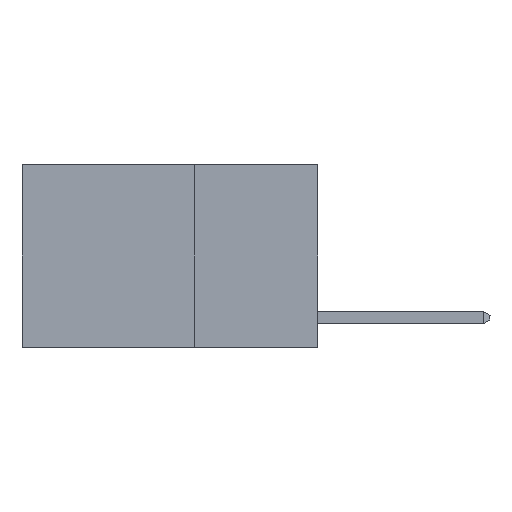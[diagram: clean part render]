
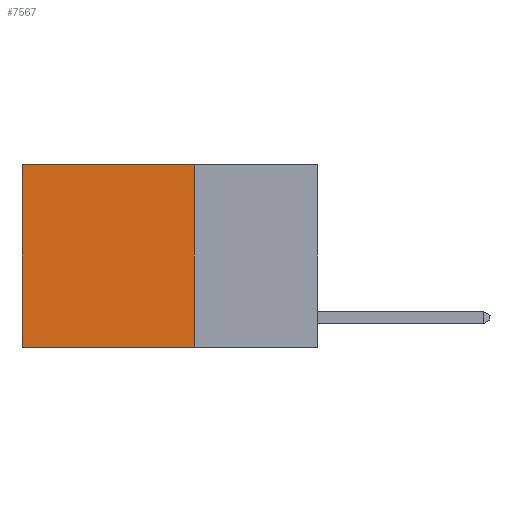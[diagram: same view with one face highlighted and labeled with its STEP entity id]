
A CAD part, left-side view. The second image highlights one B-rep face of the part: STEP entity #7567.
In plain terms, the highlighted planar face has unit normal (-1, 0, 0).
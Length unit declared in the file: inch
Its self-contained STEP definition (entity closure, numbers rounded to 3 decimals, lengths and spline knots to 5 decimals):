
#703 = AXIS2_PLACEMENT_3D ( 'NONE', #1785, #10758, #3123 ) ;
#1694 = EDGE_CURVE ( 'NONE', #4359, #4167, #3257, .T. ) ;
#1785 = CARTESIAN_POINT ( 'NONE',  ( 0.2625, 0.25, 0. ) ) ;
#1978 = CARTESIAN_POINT ( 'NONE',  ( 0.2625, 0.6, 0. ) ) ;
#2358 = VECTOR ( 'NONE', #15850, 39.37008 ) ;
#2381 = DIRECTION ( 'NONE',  ( 0., 0., -1. ) ) ;
#3123 = DIRECTION ( 'NONE',  ( 0., 0., -1. ) ) ;
#3257 = LINE ( 'NONE', #7504, #16372 ) ;
#3859 = CARTESIAN_POINT ( 'NONE',  ( 0.2625, 0.6, 0. ) ) ;
#4167 = VERTEX_POINT ( 'NONE', #13826 ) ;
#4359 = VERTEX_POINT ( 'NONE', #5326 ) ;
#4520 = FACE_OUTER_BOUND ( 'NONE', #5759, .T. ) ;
#4806 = EDGE_CURVE ( 'NONE', #4167, #10890, #10575, .T. ) ;
#5100 = EDGE_CURVE ( 'NONE', #4359, #16503, #12557, .T. ) ;
#5138 = DIRECTION ( 'NONE',  ( 0., 0., -1. ) ) ;
#5146 = CARTESIAN_POINT ( 'NONE',  ( 0.2625, 0.25, -0.37 ) ) ;
#5205 = DIRECTION ( 'NONE',  ( 0., 1., 0. ) ) ;
#5326 = CARTESIAN_POINT ( 'NONE',  ( 0.2625, 0.25, 0. ) ) ;
#5759 = EDGE_LOOP ( 'NONE', ( #6953, #8954, #7187, #14152 ) ) ;
#6166 = LINE ( 'NONE', #3859, #16259 ) ;
#6953 = ORIENTED_EDGE ( 'NONE', *, *, #12420, .T. ) ;
#6990 = CARTESIAN_POINT ( 'NONE',  ( 0.2625, 0.25, 0. ) ) ;
#7187 = ORIENTED_EDGE ( 'NONE', *, *, #1694, .F. ) ;
#7504 = CARTESIAN_POINT ( 'NONE',  ( 0.2625, 0.25, 0. ) ) ;
#7567 = ADVANCED_FACE ( 'NONE', ( #4520 ), #9465, .F. ) ;
#8954 = ORIENTED_EDGE ( 'NONE', *, *, #4806, .F. ) ;
#9465 = PLANE ( 'NONE',  #703 ) ;
#10575 = LINE ( 'NONE', #5146, #13541 ) ;
#10758 = DIRECTION ( 'NONE',  ( 1., 0., 0. ) ) ;
#10890 = VERTEX_POINT ( 'NONE', #13572 ) ;
#12420 = EDGE_CURVE ( 'NONE', #16503, #10890, #6166, .T. ) ;
#12557 = LINE ( 'NONE', #6990, #2358 ) ;
#13541 = VECTOR ( 'NONE', #5205, 39.37008 ) ;
#13572 = CARTESIAN_POINT ( 'NONE',  ( 0.2625, 0.6, -0.37 ) ) ;
#13826 = CARTESIAN_POINT ( 'NONE',  ( 0.2625, 0.25, -0.37 ) ) ;
#14152 = ORIENTED_EDGE ( 'NONE', *, *, #5100, .T. ) ;
#15850 = DIRECTION ( 'NONE',  ( 0., 1., 0. ) ) ;
#16259 = VECTOR ( 'NONE', #5138, 39.37008 ) ;
#16372 = VECTOR ( 'NONE', #2381, 39.37008 ) ;
#16503 = VERTEX_POINT ( 'NONE', #1978 ) ;
